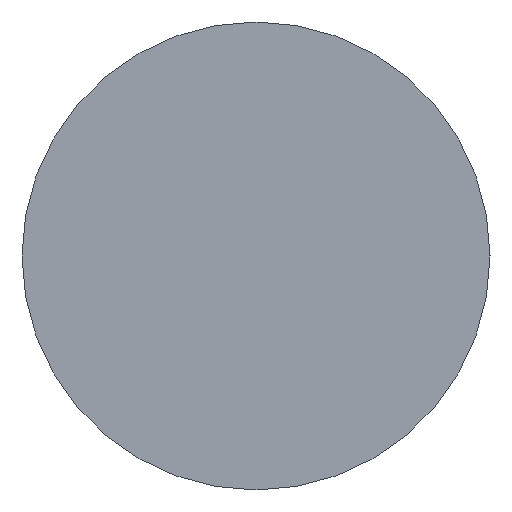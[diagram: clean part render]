
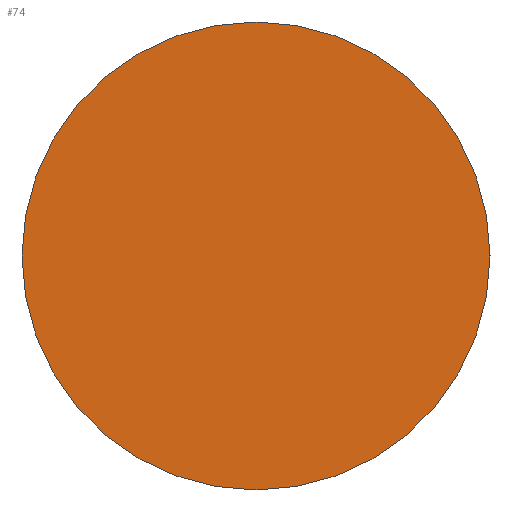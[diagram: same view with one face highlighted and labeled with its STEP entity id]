
A CAD part, left-side view. The second image highlights one B-rep face of the part: STEP entity #74.
In plain terms, the highlighted planar face has unit normal (-1, 0, 0).
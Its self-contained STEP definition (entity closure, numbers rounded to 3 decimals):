
#11 = DIRECTION ( 'NONE',  ( 1., 0., 0. ) ) ;
#13 = CARTESIAN_POINT ( 'NONE',  ( 10.625, 0., 3.75 ) ) ;
#20 = CARTESIAN_POINT ( 'NONE',  ( 10.625, 0., 0. ) ) ;
#22 = CARTESIAN_POINT ( 'NONE',  ( 10.625, 0., 0. ) ) ;
#24 = PLANE ( 'NONE',  #43 ) ;
#28 = EDGE_LOOP ( 'NONE', ( #141, #149 ) ) ;
#31 = DIRECTION ( 'NONE',  ( 1., 0., 0. ) ) ;
#43 = AXIS2_PLACEMENT_3D ( 'NONE', #20, #71, #68 ) ;
#46 = DIRECTION ( 'NONE',  ( 0., 0., -1. ) ) ;
#47 = VERTEX_POINT ( 'NONE', #69 ) ;
#49 = AXIS2_PLACEMENT_3D ( 'NONE', #63, #11, #158 ) ;
#57 = AXIS2_PLACEMENT_3D ( 'NONE', #22, #31, #46 ) ;
#58 = EDGE_CURVE ( 'NONE', #47, #122, #160, .T. ) ;
#63 = CARTESIAN_POINT ( 'NONE',  ( 10.625, 0., 0. ) ) ;
#68 = DIRECTION ( 'NONE',  ( 0., 0., -1. ) ) ;
#69 = CARTESIAN_POINT ( 'NONE',  ( 10.625, 0., -3.75 ) ) ;
#71 = DIRECTION ( 'NONE',  ( 1., 0., 0. ) ) ;
#72 = EDGE_CURVE ( 'NONE', #122, #47, #139, .T. ) ;
#74 = ADVANCED_FACE ( 'NONE', ( #125 ), #24, .F. ) ;
#122 = VERTEX_POINT ( 'NONE', #13 ) ;
#125 = FACE_OUTER_BOUND ( 'NONE', #28, .T. ) ;
#139 = CIRCLE ( 'NONE', #49, 3.75 ) ;
#141 = ORIENTED_EDGE ( 'NONE', *, *, #72, .F. ) ;
#149 = ORIENTED_EDGE ( 'NONE', *, *, #58, .F. ) ;
#158 = DIRECTION ( 'NONE',  ( 0., 0., -1. ) ) ;
#160 = CIRCLE ( 'NONE', #57, 3.75 ) ;
